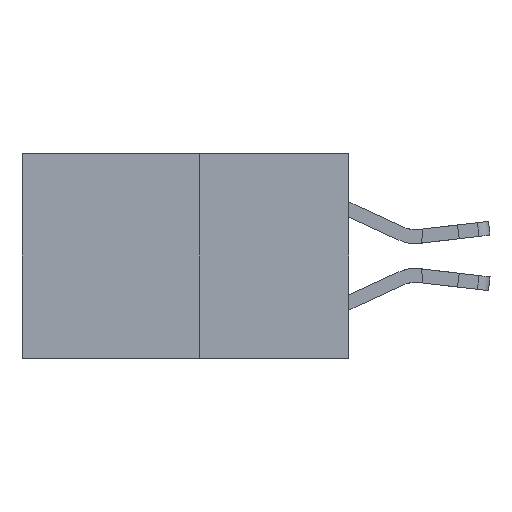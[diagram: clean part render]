
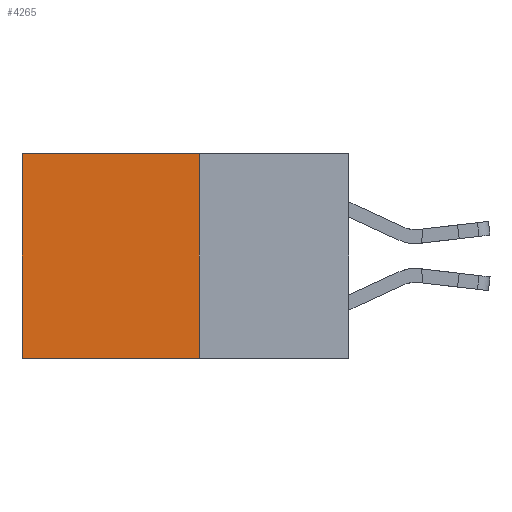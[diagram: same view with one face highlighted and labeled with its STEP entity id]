
A CAD part, left-side view. The second image highlights one B-rep face of the part: STEP entity #4265.
In plain terms, the highlighted planar face has unit normal (-1, 0, 0).
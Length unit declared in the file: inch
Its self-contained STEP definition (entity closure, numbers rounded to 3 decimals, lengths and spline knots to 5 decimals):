
#13 = CARTESIAN_POINT ( 'NONE',  ( 0.277, 0.59, -0.37 ) ) ;
#154 = DIRECTION ( 'NONE',  ( 0., 1., 0. ) ) ;
#1220 = DIRECTION ( 'NONE',  ( 0., 0., -1. ) ) ;
#1277 = DIRECTION ( 'NONE',  ( 0., 0., -1. ) ) ;
#1687 = VECTOR ( 'NONE', #14494, 39.37008 ) ;
#1915 = LINE ( 'NONE', #7671, #14391 ) ;
#3930 = LINE ( 'NONE', #6156, #13103 ) ;
#3962 = VERTEX_POINT ( 'NONE', #7144 ) ;
#4265 = ADVANCED_FACE ( 'NONE', ( #10531 ), #7225, .F. ) ;
#4289 = CARTESIAN_POINT ( 'NONE',  ( 0.277, 0.27, -0.37 ) ) ;
#4594 = CARTESIAN_POINT ( 'NONE',  ( 0.277, 0.27, 0. ) ) ;
#5124 = VERTEX_POINT ( 'NONE', #4594 ) ;
#5956 = DIRECTION ( 'NONE',  ( 1., 0., 0. ) ) ;
#6143 = CARTESIAN_POINT ( 'NONE',  ( 0.277, 0.27, 0. ) ) ;
#6156 = CARTESIAN_POINT ( 'NONE',  ( 0.277, 0.27, -0.37 ) ) ;
#6210 = ORIENTED_EDGE ( 'NONE', *, *, #6379, .F. ) ;
#6379 = EDGE_CURVE ( 'NONE', #5124, #10428, #1915, .T. ) ;
#6597 = DIRECTION ( 'NONE',  ( 0., 0., -1. ) ) ;
#7144 = CARTESIAN_POINT ( 'NONE',  ( 0.277, 0.59, -0.37 ) ) ;
#7208 = EDGE_CURVE ( 'NONE', #11233, #3962, #7818, .T. ) ;
#7225 = PLANE ( 'NONE',  #11759 ) ;
#7671 = CARTESIAN_POINT ( 'NONE',  ( 0.277, 0.27, -0.37 ) ) ;
#7793 = LINE ( 'NONE', #6143, #1687 ) ;
#7818 = LINE ( 'NONE', #13, #10655 ) ;
#8565 = EDGE_LOOP ( 'NONE', ( #10157, #12560, #6210, #9015 ) ) ;
#8731 = EDGE_CURVE ( 'NONE', #5124, #11233, #7793, .T. ) ;
#8854 = CARTESIAN_POINT ( 'NONE',  ( 0.277, 0.59, 0. ) ) ;
#9015 = ORIENTED_EDGE ( 'NONE', *, *, #8731, .T. ) ;
#9155 = CARTESIAN_POINT ( 'NONE',  ( 0.277, 0.27, -0.37 ) ) ;
#10157 = ORIENTED_EDGE ( 'NONE', *, *, #7208, .T. ) ;
#10428 = VERTEX_POINT ( 'NONE', #4289 ) ;
#10531 = FACE_OUTER_BOUND ( 'NONE', #8565, .T. ) ;
#10655 = VECTOR ( 'NONE', #1220, 39.37008 ) ;
#11233 = VERTEX_POINT ( 'NONE', #8854 ) ;
#11759 = AXIS2_PLACEMENT_3D ( 'NONE', #9155, #5956, #1277 ) ;
#12560 = ORIENTED_EDGE ( 'NONE', *, *, #12771, .F. ) ;
#12771 = EDGE_CURVE ( 'NONE', #10428, #3962, #3930, .T. ) ;
#13103 = VECTOR ( 'NONE', #154, 39.37008 ) ;
#14391 = VECTOR ( 'NONE', #6597, 39.37008 ) ;
#14494 = DIRECTION ( 'NONE',  ( 0., 1., 0. ) ) ;
